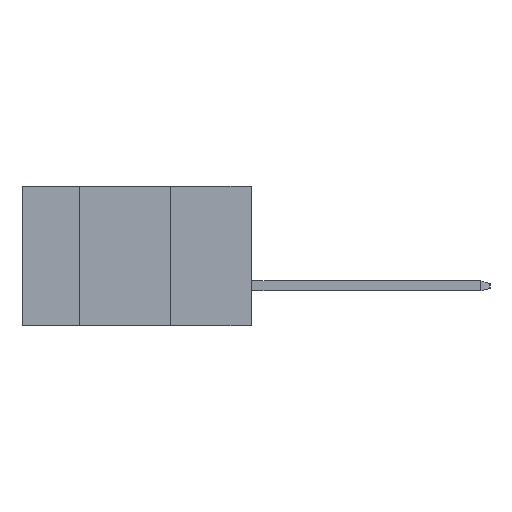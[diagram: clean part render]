
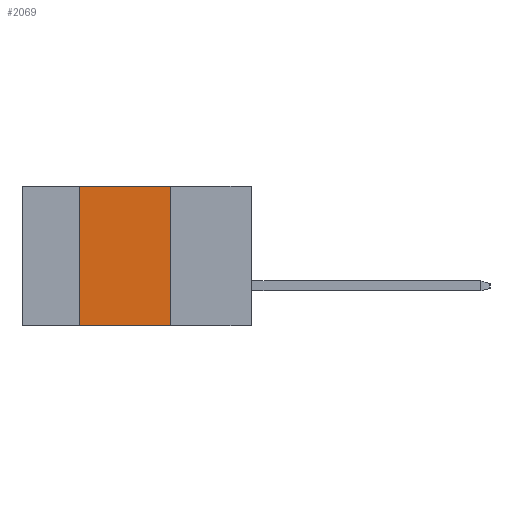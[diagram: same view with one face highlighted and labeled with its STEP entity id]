
A CAD part, left-side view. The second image highlights one B-rep face of the part: STEP entity #2069.
In plain terms, the highlighted planar face has unit normal (-1, 0, 0).
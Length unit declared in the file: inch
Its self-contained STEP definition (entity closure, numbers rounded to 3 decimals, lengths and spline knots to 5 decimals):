
#279 = VERTEX_POINT ( 'NONE', #4549 ) ;
#347 = AXIS2_PLACEMENT_3D ( 'NONE', #631, #838, #8334 ) ;
#425 = CARTESIAN_POINT ( 'NONE',  ( 0., 0.54, 0. ) ) ;
#535 = EDGE_CURVE ( 'NONE', #3237, #5833, #5639, .T. ) ;
#631 = CARTESIAN_POINT ( 'NONE',  ( 0., 0.72, 0. ) ) ;
#838 = DIRECTION ( 'NONE',  ( 1., 0., 0. ) ) ;
#1208 = EDGE_CURVE ( 'NONE', #5321, #279, #3274, .T. ) ;
#1477 = DIRECTION ( 'NONE',  ( 0., 0., 1. ) ) ;
#1517 = DIRECTION ( 'NONE',  ( 0., -1., 0. ) ) ;
#1560 = CARTESIAN_POINT ( 'NONE',  ( 0., 0.72, -0.437 ) ) ;
#1880 = VECTOR ( 'NONE', #1477, 39.37008 ) ;
#2046 = CARTESIAN_POINT ( 'NONE',  ( 0., 0.72, 0. ) ) ;
#2069 = ADVANCED_FACE ( 'NONE', ( #6474 ), #4128, .F. ) ;
#2264 = EDGE_CURVE ( 'NONE', #5833, #5321, #7076, .T. ) ;
#2366 = ORIENTED_EDGE ( 'NONE', *, *, #1208, .F. ) ;
#2626 = VECTOR ( 'NONE', #1517, 39.37008 ) ;
#2729 = CARTESIAN_POINT ( 'NONE',  ( 0., 0.254, 0. ) ) ;
#2942 = EDGE_CURVE ( 'NONE', #3237, #279, #7357, .T. ) ;
#3237 = VERTEX_POINT ( 'NONE', #10405 ) ;
#3274 = LINE ( 'NONE', #5784, #7655 ) ;
#3391 = DIRECTION ( 'NONE',  ( 0., 0., -1. ) ) ;
#4128 = PLANE ( 'NONE',  #347 ) ;
#4549 = CARTESIAN_POINT ( 'NONE',  ( 0., 0.254, -0.437 ) ) ;
#4787 = EDGE_LOOP ( 'NONE', ( #2366, #5655, #4951, #8878 ) ) ;
#4951 = ORIENTED_EDGE ( 'NONE', *, *, #535, .F. ) ;
#5321 = VERTEX_POINT ( 'NONE', #2729 ) ;
#5639 = LINE ( 'NONE', #8980, #1880 ) ;
#5655 = ORIENTED_EDGE ( 'NONE', *, *, #2264, .F. ) ;
#5784 = CARTESIAN_POINT ( 'NONE',  ( 0., 0.254, -0.437 ) ) ;
#5833 = VERTEX_POINT ( 'NONE', #425 ) ;
#6474 = FACE_OUTER_BOUND ( 'NONE', #4787, .T. ) ;
#7076 = LINE ( 'NONE', #2046, #2626 ) ;
#7357 = LINE ( 'NONE', #1560, #9607 ) ;
#7655 = VECTOR ( 'NONE', #3391, 39.37008 ) ;
#8334 = DIRECTION ( 'NONE',  ( 0., 0., -1. ) ) ;
#8878 = ORIENTED_EDGE ( 'NONE', *, *, #2942, .T. ) ;
#8980 = CARTESIAN_POINT ( 'NONE',  ( 0., 0.54, -0.437 ) ) ;
#9216 = DIRECTION ( 'NONE',  ( 0., -1., 0. ) ) ;
#9607 = VECTOR ( 'NONE', #9216, 39.37008 ) ;
#10405 = CARTESIAN_POINT ( 'NONE',  ( 0., 0.54, -0.437 ) ) ;
